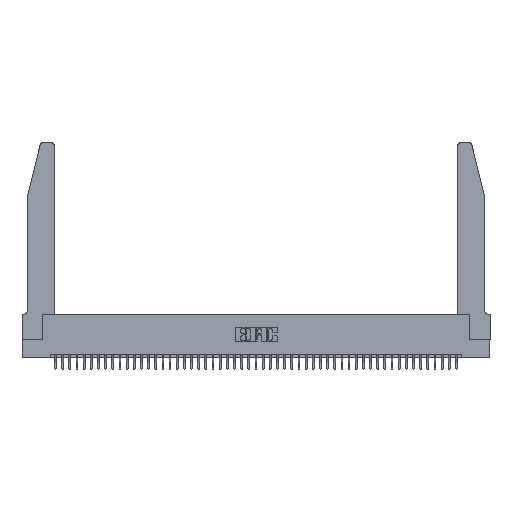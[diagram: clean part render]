
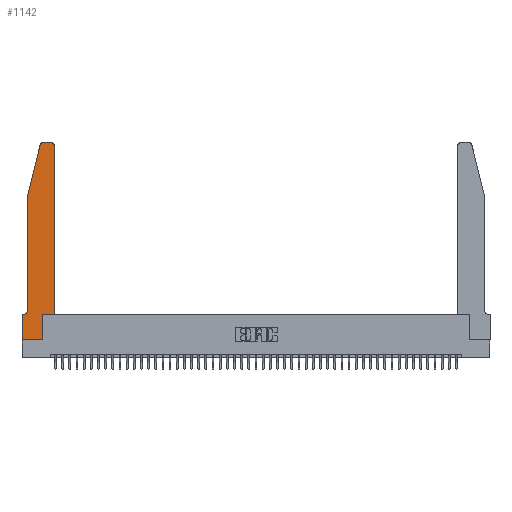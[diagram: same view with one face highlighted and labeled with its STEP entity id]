
A CAD part, top view. The second image highlights one B-rep face of the part: STEP entity #1142.
In plain terms, the highlighted planar face has unit normal (0, 0, 1).
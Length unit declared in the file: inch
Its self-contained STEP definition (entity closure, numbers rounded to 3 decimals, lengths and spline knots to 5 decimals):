
#443 = EDGE_CURVE ( 'NONE', #14354, #4320, #23194, .T. ) ;
#457 = VECTOR ( 'NONE', #46939, 39.37008 ) ;
#464 = DIRECTION ( 'NONE',  ( 0., 0., 1. ) ) ;
#513 = LINE ( 'NONE', #19805, #38622 ) ;
#1142 = ADVANCED_FACE ( 'NONE', ( #40488 ), #8939, .T. ) ;
#3404 = CARTESIAN_POINT ( 'NONE',  ( 0.4505, 0.35, 0.37 ) ) ;
#3572 = DIRECTION ( 'NONE',  ( 0., 0., -1. ) ) ;
#4320 = VERTEX_POINT ( 'NONE', #47089 ) ;
#6113 = VERTEX_POINT ( 'NONE', #29328 ) ;
#6295 = ORIENTED_EDGE ( 'NONE', *, *, #39482, .T. ) ;
#6914 = VECTOR ( 'NONE', #40387, 39.37008 ) ;
#6970 = VECTOR ( 'NONE', #46189, 39.37008 ) ;
#7017 = LINE ( 'NONE', #21605, #8155 ) ;
#7196 = ORIENTED_EDGE ( 'NONE', *, *, #17244, .T. ) ;
#7254 = ORIENTED_EDGE ( 'NONE', *, *, #40257, .T. ) ;
#7453 = ORIENTED_EDGE ( 'NONE', *, *, #34928, .T. ) ;
#7599 = VECTOR ( 'NONE', #33432, 39.37008 ) ;
#7608 = CARTESIAN_POINT ( 'NONE',  ( 0., 0., 0.37 ) ) ;
#8155 = VECTOR ( 'NONE', #29021, 39.37008 ) ;
#8789 = AXIS2_PLACEMENT_3D ( 'NONE', #22522, #464, #22684 ) ;
#8939 = PLANE ( 'NONE',  #9207 ) ;
#8957 = VERTEX_POINT ( 'NONE', #46077 ) ;
#9207 = AXIS2_PLACEMENT_3D ( 'NONE', #43255, #17814, #29279 ) ;
#10251 = LINE ( 'NONE', #3404, #457 ) ;
#11034 = CARTESIAN_POINT ( 'NONE',  ( 0.0755, 2., 0.37 ) ) ;
#11186 = VERTEX_POINT ( 'NONE', #44193 ) ;
#12087 = LINE ( 'NONE', #30795, #46168 ) ;
#12383 = DIRECTION ( 'NONE',  ( 0., 1., 0. ) ) ;
#12472 = CARTESIAN_POINT ( 'NONE',  ( 0., 0., 0.37 ) ) ;
#14353 = ORIENTED_EDGE ( 'NONE', *, *, #40259, .T. ) ;
#14354 = VERTEX_POINT ( 'NONE', #28729 ) ;
#17244 = EDGE_CURVE ( 'NONE', #18787, #28200, #31180, .T. ) ;
#17324 = LINE ( 'NONE', #12472, #6970 ) ;
#17545 = CARTESIAN_POINT ( 'NONE',  ( 0.2865, 0., 0.37 ) ) ;
#17638 = VERTEX_POINT ( 'NONE', #35531 ) ;
#17749 = EDGE_CURVE ( 'NONE', #31728, #11186, #23613, .T. ) ;
#17814 = DIRECTION ( 'NONE',  ( 0., 0., 1. ) ) ;
#18097 = AXIS2_PLACEMENT_3D ( 'NONE', #47405, #3572, #47256 ) ;
#18787 = VERTEX_POINT ( 'NONE', #35404 ) ;
#19570 = EDGE_CURVE ( 'NONE', #6113, #8957, #10251, .T. ) ;
#19805 = CARTESIAN_POINT ( 'NONE',  ( 0.0755, 2., 0.37 ) ) ;
#21030 = ORIENTED_EDGE ( 'NONE', *, *, #443, .T. ) ;
#21605 = CARTESIAN_POINT ( 'NONE',  ( 0.4505, 0.35, 0.37 ) ) ;
#21984 = DIRECTION ( 'NONE',  ( 0., 0., 1. ) ) ;
#22522 = CARTESIAN_POINT ( 'NONE',  ( 0.4205, 2.72, 0.37 ) ) ;
#22684 = DIRECTION ( 'NONE',  ( 1., 0., 0. ) ) ;
#23194 = LINE ( 'NONE', #43177, #42817 ) ;
#23201 = EDGE_CURVE ( 'NONE', #36923, #31728, #513, .T. ) ;
#23239 = VECTOR ( 'NONE', #46893, 39.37008 ) ;
#23613 = CIRCLE ( 'NONE', #18097, 0.07 ) ;
#24336 = DIRECTION ( 'NONE',  ( -1., 0., 0. ) ) ;
#25857 = CARTESIAN_POINT ( 'NONE',  ( 0.0755, 0.42, 0.37 ) ) ;
#27252 = LINE ( 'NONE', #40549, #7599 ) ;
#27887 = ORIENTED_EDGE ( 'NONE', *, *, #23201, .T. ) ;
#28200 = VERTEX_POINT ( 'NONE', #17545 ) ;
#28441 = LINE ( 'NONE', #39343, #23239 ) ;
#28729 = CARTESIAN_POINT ( 'NONE',  ( 0.4205, 2.75, 0.37 ) ) ;
#29021 = DIRECTION ( 'NONE',  ( 1., 0., 0. ) ) ;
#29245 = DIRECTION ( 'NONE',  ( 1., 0., 0. ) ) ;
#29279 = DIRECTION ( 'NONE',  ( 1., 0., 0. ) ) ;
#29328 = CARTESIAN_POINT ( 'NONE',  ( 0.4505, 0.35, 0.37 ) ) ;
#30228 = CARTESIAN_POINT ( 'NONE',  ( 0., 0.35, 0.37 ) ) ;
#30795 = CARTESIAN_POINT ( 'NONE',  ( 0.2865, 0.35, 0.37 ) ) ;
#30914 = ORIENTED_EDGE ( 'NONE', *, *, #19570, .T. ) ;
#31030 = ORIENTED_EDGE ( 'NONE', *, *, #17749, .T. ) ;
#31180 = LINE ( 'NONE', #7608, #6914 ) ;
#31728 = VERTEX_POINT ( 'NONE', #25857 ) ;
#32050 = ORIENTED_EDGE ( 'NONE', *, *, #45844, .T. ) ;
#32780 = EDGE_CURVE ( 'NONE', #37143, #18787, #17324, .T. ) ;
#33432 = DIRECTION ( 'NONE',  ( -0.239, -0.971, 0. ) ) ;
#34490 = DIRECTION ( 'NONE',  ( 0., -1., 0. ) ) ;
#34928 = EDGE_CURVE ( 'NONE', #8957, #14354, #36234, .T. ) ;
#35404 = CARTESIAN_POINT ( 'NONE',  ( 0., 0., 0.37 ) ) ;
#35531 = CARTESIAN_POINT ( 'NONE',  ( 0.25487, 2.72718, 0.37 ) ) ;
#36234 = CIRCLE ( 'NONE', #8789, 0.03 ) ;
#36923 = VERTEX_POINT ( 'NONE', #11034 ) ;
#37143 = VERTEX_POINT ( 'NONE', #30228 ) ;
#37450 = ORIENTED_EDGE ( 'NONE', *, *, #32780, .T. ) ;
#38353 = ORIENTED_EDGE ( 'NONE', *, *, #41137, .T. ) ;
#38622 = VECTOR ( 'NONE', #34490, 39.37008 ) ;
#39343 = CARTESIAN_POINT ( 'NONE',  ( 0.0755, 0.35, 0.37 ) ) ;
#39482 = EDGE_CURVE ( 'NONE', #11186, #37143, #28441, .T. ) ;
#40257 = EDGE_CURVE ( 'NONE', #17638, #36923, #27252, .T. ) ;
#40259 = EDGE_CURVE ( 'NONE', #4320, #17638, #45085, .T. ) ;
#40387 = DIRECTION ( 'NONE',  ( 1., 0., 0. ) ) ;
#40488 = FACE_OUTER_BOUND ( 'NONE', #45851, .T. ) ;
#40549 = CARTESIAN_POINT ( 'NONE',  ( 0.0755, 2., 0.37 ) ) ;
#40598 = AXIS2_PLACEMENT_3D ( 'NONE', #44381, #21984, #29245 ) ;
#41137 = EDGE_CURVE ( 'NONE', #28200, #46227, #12087, .T. ) ;
#42817 = VECTOR ( 'NONE', #24336, 39.37008 ) ;
#43177 = CARTESIAN_POINT ( 'NONE',  ( 0.2605, 2.75, 0.37 ) ) ;
#43255 = CARTESIAN_POINT ( 'NONE',  ( 0., 0.35, 0.37 ) ) ;
#44193 = CARTESIAN_POINT ( 'NONE',  ( 0.0055, 0.35, 0.37 ) ) ;
#44381 = CARTESIAN_POINT ( 'NONE',  ( 0.284, 2.72, 0.37 ) ) ;
#45085 = CIRCLE ( 'NONE', #40598, 0.03 ) ;
#45844 = EDGE_CURVE ( 'NONE', #46227, #6113, #7017, .T. ) ;
#45851 = EDGE_LOOP ( 'NONE', ( #21030, #14353, #7254, #27887, #31030, #6295, #37450, #7196, #38353, #32050, #30914, #7453 ) ) ;
#46076 = CARTESIAN_POINT ( 'NONE',  ( 0.2865, 0.35, 0.37 ) ) ;
#46077 = CARTESIAN_POINT ( 'NONE',  ( 0.4505, 2.72, 0.37 ) ) ;
#46168 = VECTOR ( 'NONE', #12383, 39.37008 ) ;
#46189 = DIRECTION ( 'NONE',  ( 0., -1., 0. ) ) ;
#46227 = VERTEX_POINT ( 'NONE', #46076 ) ;
#46893 = DIRECTION ( 'NONE',  ( -1., 0., 0. ) ) ;
#46939 = DIRECTION ( 'NONE',  ( 0., 1., 0. ) ) ;
#47089 = CARTESIAN_POINT ( 'NONE',  ( 0.284, 2.75, 0.37 ) ) ;
#47256 = DIRECTION ( 'NONE',  ( -1., 0., 0. ) ) ;
#47405 = CARTESIAN_POINT ( 'NONE',  ( 0.0055, 0.42, 0.37 ) ) ;
